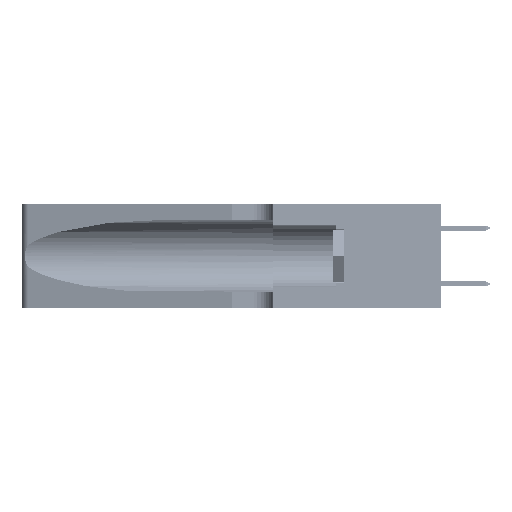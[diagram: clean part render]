
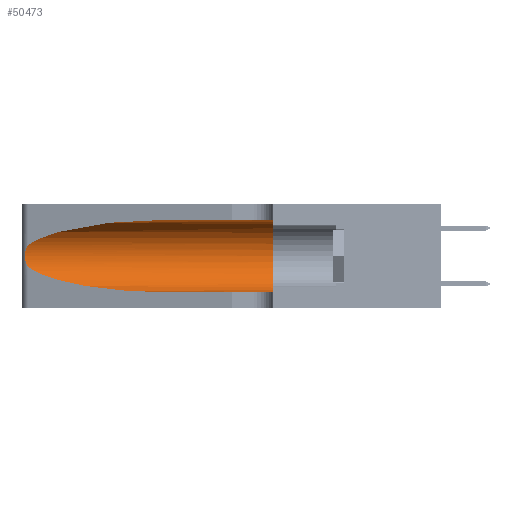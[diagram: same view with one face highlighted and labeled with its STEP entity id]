
A CAD part, left-side view. The second image highlights one B-rep face of the part: STEP entity #50473.
In plain terms, the highlighted cylindrical face has radius 3.308 mm (diameter 6.617 mm), a partial arc.
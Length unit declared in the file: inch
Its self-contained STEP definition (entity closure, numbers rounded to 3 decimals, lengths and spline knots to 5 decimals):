
#246 = CARTESIAN_POINT ( 'NONE',  ( 0.18966, 0.96281, 0.05475 ) ) ;
#247 = AXIS2_PLACEMENT_3D ( 'NONE', #19702, #44902, #19516 ) ;
#2289 = FACE_OUTER_BOUND ( 'NONE', #41994, .T. ) ;
#2732 = ORIENTED_EDGE ( 'NONE', *, *, #20181, .T. ) ;
#2911 = CARTESIAN_POINT ( 'NONE',  ( 0.1305, 0.35, 0.05475 ) ) ;
#3454 = CARTESIAN_POINT ( 'NONE',  ( 0.25789, 1.23486, 0.15765 ) ) ;
#6187 =( BOUNDED_CURVE ( )  B_SPLINE_CURVE ( 3, ( #29417, #33610, #50370, #25578 ),
 .UNSPECIFIED., .F., .F. ) 
 B_SPLINE_CURVE_WITH_KNOTS ( ( 4, 4 ),
 ( 1.5708, 2.84003 ),
 .UNSPECIFIED. ) 
 CURVE ( )  GEOMETRIC_REPRESENTATION_ITEM ( )  RATIONAL_B_SPLINE_CURVE ( ( 1., 0.87, 0.87, 1. ) ) 
 REPRESENTATION_ITEM ( '' )  );
#6495 = CIRCLE ( 'NONE', #247, 0.13025 ) ;
#7094 = EDGE_CURVE ( 'NONE', #8681, #46417, #6187, .T. ) ;
#7178 = LINE ( 'NONE', #53078, #20327 ) ;
#7634 = CARTESIAN_POINT ( 'NONE',  ( 0.25487, 1.22718, 0.14631 ) ) ;
#8681 = VERTEX_POINT ( 'NONE', #21598 ) ;
#8746 = LINE ( 'NONE', #22088, #24444 ) ;
#9250 = DIRECTION ( 'NONE',  ( 0., -1., 0. ) ) ;
#12011 = CARTESIAN_POINT ( 'NONE',  ( 0.26075, 1.23896, 0.19203 ) ) ;
#12357 = CARTESIAN_POINT ( 'NONE',  ( 0.25487, 1.22718, 0.22369 ) ) ;
#13354 = CARTESIAN_POINT ( 'NONE',  ( 0.25487, 1.22718, 0.14631 ) ) ;
#13465 = DIRECTION ( 'NONE',  ( 0., 0., -1. ) ) ;
#14034 = ORIENTED_EDGE ( 'NONE', *, *, #47175, .F. ) ;
#14170 = VERTEX_POINT ( 'NONE', #2911 ) ;
#15884 = CARTESIAN_POINT ( 'NONE',  ( 0.26017, 1.23833, 0.17102 ) ) ;
#16240 = CARTESIAN_POINT ( 'NONE',  ( 0.25639, 1.23186, 0.15144 ) ) ;
#16530 = CARTESIAN_POINT ( 'NONE',  ( 0.25487, 1.22718, 0.14631 ) ) ;
#16594 = CARTESIAN_POINT ( 'NONE',  ( 0.26018, 1.23835, 0.19895 ) ) ;
#16968 = CARTESIAN_POINT ( 'NONE',  ( 0.1305, 1.61858, 0.185 ) ) ;
#17060 = CARTESIAN_POINT ( 'NONE',  ( 0.1305, 0.72297, 0.05475 ) ) ;
#18130 = CARTESIAN_POINT ( 'NONE',  ( 0.1305, 0.72297, 0.05475 ) ) ;
#19516 = DIRECTION ( 'NONE',  ( 0., 0., 1. ) ) ;
#19702 = CARTESIAN_POINT ( 'NONE',  ( 0.1305, 0.35, 0.185 ) ) ;
#20181 = EDGE_CURVE ( 'NONE', #30043, #41953, #31327, .T. ) ;
#20327 = VECTOR ( 'NONE', #48853, 39.37008 ) ;
#21435 = CARTESIAN_POINT ( 'NONE',  ( 0.25854, 1.2359, 0.20912 ) ) ;
#21598 = CARTESIAN_POINT ( 'NONE',  ( 0.1305, 0.72297, 0.31525 ) ) ;
#22088 = CARTESIAN_POINT ( 'NONE',  ( 0.1305, 1.61858, 0.05475 ) ) ;
#24380 = VERTEX_POINT ( 'NONE', #38325 ) ;
#24444 = VECTOR ( 'NONE', #47417, 39.37008 ) ;
#25578 = CARTESIAN_POINT ( 'NONE',  ( 0.25487, 1.22718, 0.22369 ) ) ;
#28659 = CARTESIAN_POINT ( 'NONE',  ( 0.25787, 1.23484, 0.2124 ) ) ;
#29066 = EDGE_CURVE ( 'NONE', #8681, #24380, #7178, .T. ) ;
#29417 = CARTESIAN_POINT ( 'NONE',  ( 0.1305, 0.72297, 0.31525 ) ) ;
#30043 = VERTEX_POINT ( 'NONE', #13354 ) ;
#31327 =( BOUNDED_CURVE ( )  B_SPLINE_CURVE ( 3, ( #16530, #37334, #246, #17060 ),
 .UNSPECIFIED., .F., .F. ) 
 B_SPLINE_CURVE_WITH_KNOTS ( ( 4, 4 ),
 ( 3.44316, 4.71239 ),
 .UNSPECIFIED. ) 
 CURVE ( )  GEOMETRIC_REPRESENTATION_ITEM ( )  RATIONAL_B_SPLINE_CURVE ( ( 1., 0.87, 0.87, 1. ) ) 
 REPRESENTATION_ITEM ( '' )  );
#32499 = CARTESIAN_POINT ( 'NONE',  ( 0.25555, 1.22994, 0.2215 ) ) ;
#32681 = CARTESIAN_POINT ( 'NONE',  ( 0.25555, 1.22993, 0.14849 ) ) ;
#33009 = CYLINDRICAL_SURFACE ( 'NONE', #51590, 0.13025 ) ;
#33039 = ORIENTED_EDGE ( 'NONE', *, *, #7094, .T. ) ;
#33610 = CARTESIAN_POINT ( 'NONE',  ( 0.18966, 0.96281, 0.31525 ) ) ;
#33985 = ORIENTED_EDGE ( 'NONE', *, *, #36708, .T. ) ;
#36708 = EDGE_CURVE ( 'NONE', #41953, #14170, #8746, .T. ) ;
#37334 = CARTESIAN_POINT ( 'NONE',  ( 0.2373, 1.15595, 0.08982 ) ) ;
#38325 = CARTESIAN_POINT ( 'NONE',  ( 0.1305, 0.35, 0.31525 ) ) ;
#41256 = CARTESIAN_POINT ( 'NONE',  ( 0.26075, 1.23896, 0.178 ) ) ;
#41953 = VERTEX_POINT ( 'NONE', #18130 ) ;
#41994 = EDGE_LOOP ( 'NONE', ( #33039, #42677, #2732, #33985, #14034, #52409 ) ) ;
#42677 = ORIENTED_EDGE ( 'NONE', *, *, #43940, .T. ) ;
#43940 = EDGE_CURVE ( 'NONE', #46417, #30043, #50685, .T. ) ;
#44439 = CARTESIAN_POINT ( 'NONE',  ( 0.25487, 1.22718, 0.22369 ) ) ;
#44902 = DIRECTION ( 'NONE',  ( 0., 1., 0. ) ) ;
#46417 = VERTEX_POINT ( 'NONE', #44439 ) ;
#47175 = EDGE_CURVE ( 'NONE', #24380, #14170, #6495, .T. ) ;
#47417 = DIRECTION ( 'NONE',  ( 0., -1., 0. ) ) ;
#48853 = DIRECTION ( 'NONE',  ( 0., -1., 0. ) ) ;
#49261 = CARTESIAN_POINT ( 'NONE',  ( 0.25856, 1.23593, 0.16098 ) ) ;
#49456 = CARTESIAN_POINT ( 'NONE',  ( 0.25639, 1.23184, 0.21858 ) ) ;
#50370 = CARTESIAN_POINT ( 'NONE',  ( 0.2373, 1.15595, 0.28018 ) ) ;
#50473 = ADVANCED_FACE ( 'NONE', ( #2289 ), #33009, .F. ) ;
#50685 = B_SPLINE_CURVE_WITH_KNOTS ( 'NONE', 3,
 ( #12357, #32499, #49456, #28659, #21435, #16594, #12011, #41256, #15884, #49261, #3454, #16240, #32681, #7634 ),
 .UNSPECIFIED., .F., .F.,
 ( 4, 2, 2, 2, 2, 2, 4 ),
 ( 0., 0.00027, 0.00053, 0.00107, 0.0016, 0.00187, 0.00214 ),
 .UNSPECIFIED. ) ;
#51590 = AXIS2_PLACEMENT_3D ( 'NONE', #16968, #9250, #13465 ) ;
#52409 = ORIENTED_EDGE ( 'NONE', *, *, #29066, .F. ) ;
#53078 = CARTESIAN_POINT ( 'NONE',  ( 0.1305, 1.61858, 0.31525 ) ) ;
